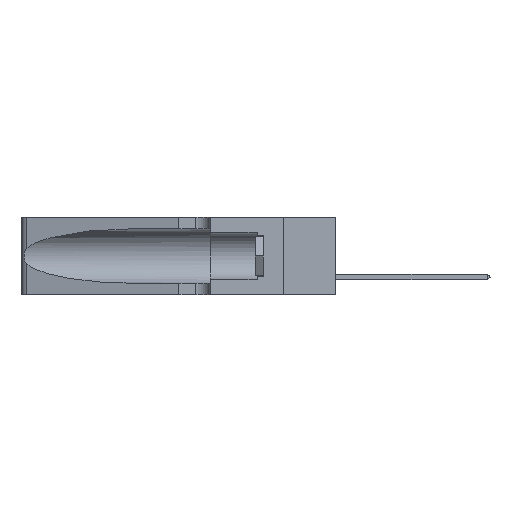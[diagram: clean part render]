
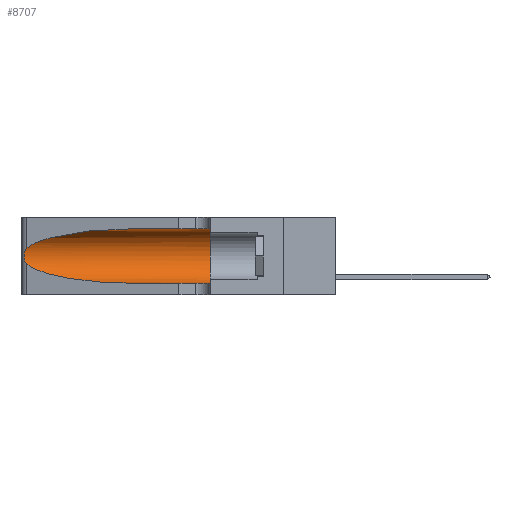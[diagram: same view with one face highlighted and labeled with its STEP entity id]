
A CAD part, left-side view. The second image highlights one B-rep face of the part: STEP entity #8707.
In plain terms, the highlighted cylindrical face has radius 3.308 mm (diameter 6.617 mm), a partial arc.
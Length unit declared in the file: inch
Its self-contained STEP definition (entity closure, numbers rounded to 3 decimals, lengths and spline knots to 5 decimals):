
#660 = EDGE_CURVE ( 'NONE', #13352, #8975, #31442, .T. ) ;
#993 = CARTESIAN_POINT ( 'NONE',  ( 0.25789, 1.23486, 0.15765 ) ) ;
#1196 = EDGE_CURVE ( 'NONE', #33338, #35989, #2201, .T. ) ;
#2098 = CARTESIAN_POINT ( 'NONE',  ( 0.25487, 1.22718, 0.22369 ) ) ;
#2140 = DIRECTION ( 'NONE',  ( 0., 0., -1. ) ) ;
#2201 =( BOUNDED_CURVE ( )  B_SPLINE_CURVE ( 3, ( #18790, #30585, #4797, #10540 ),
 .UNSPECIFIED., .F., .F. ) 
 B_SPLINE_CURVE_WITH_KNOTS ( ( 4, 4 ),
 ( 1.5708, 2.84003 ),
 .UNSPECIFIED. ) 
 CURVE ( )  GEOMETRIC_REPRESENTATION_ITEM ( )  RATIONAL_B_SPLINE_CURVE ( ( 1., 0.87, 0.87, 1. ) ) 
 REPRESENTATION_ITEM ( '' )  );
#2909 = CARTESIAN_POINT ( 'NONE',  ( 0.25487, 1.22718, 0.14631 ) ) ;
#3874 = DIRECTION ( 'NONE',  ( 0., -1., 0. ) ) ;
#4797 = CARTESIAN_POINT ( 'NONE',  ( 0.2373, 1.15595, 0.28018 ) ) ;
#5353 = CARTESIAN_POINT ( 'NONE',  ( 0.1305, 0.35, 0.185 ) ) ;
#6869 = CARTESIAN_POINT ( 'NONE',  ( 0.25639, 1.23186, 0.15144 ) ) ;
#6908 = VECTOR ( 'NONE', #3874, 39.37008 ) ;
#7624 = CARTESIAN_POINT ( 'NONE',  ( 0.1305, 1.61858, 0.185 ) ) ;
#8354 = CARTESIAN_POINT ( 'NONE',  ( 0.1305, 0.35, 0.31525 ) ) ;
#8707 = ADVANCED_FACE ( 'NONE', ( #20931 ), #25402, .F. ) ;
#8975 = VERTEX_POINT ( 'NONE', #16014 ) ;
#10086 = CARTESIAN_POINT ( 'NONE',  ( 0.26075, 1.23896, 0.19203 ) ) ;
#10387 = VERTEX_POINT ( 'NONE', #24492 ) ;
#10540 = CARTESIAN_POINT ( 'NONE',  ( 0.25487, 1.22718, 0.22369 ) ) ;
#12461 =( BOUNDED_CURVE ( )  B_SPLINE_CURVE ( 3, ( #2909, #19543, #14164, #17141 ),
 .UNSPECIFIED., .F., .T. ) 
 B_SPLINE_CURVE_WITH_KNOTS ( ( 4, 4 ),
 ( 3.44316, 4.71239 ),
 .UNSPECIFIED. ) 
 CURVE ( )  GEOMETRIC_REPRESENTATION_ITEM ( )  RATIONAL_B_SPLINE_CURVE ( ( 1., 0.87, 0.87, 1. ) ) 
 REPRESENTATION_ITEM ( '' )  );
#12479 = CARTESIAN_POINT ( 'NONE',  ( 0.25639, 1.23184, 0.21858 ) ) ;
#12591 = LINE ( 'NONE', #23389, #27291 ) ;
#12749 = CARTESIAN_POINT ( 'NONE',  ( 0.1305, 1.61858, 0.31525 ) ) ;
#12853 = CARTESIAN_POINT ( 'NONE',  ( 0.25487, 1.22718, 0.22369 ) ) ;
#12978 = CARTESIAN_POINT ( 'NONE',  ( 0.26017, 1.23833, 0.17102 ) ) ;
#13092 = ORIENTED_EDGE ( 'NONE', *, *, #27038, .T. ) ;
#13352 = VERTEX_POINT ( 'NONE', #8354 ) ;
#13659 = EDGE_CURVE ( 'NONE', #33338, #13352, #21161, .T. ) ;
#14137 = ORIENTED_EDGE ( 'NONE', *, *, #13659, .F. ) ;
#14164 = CARTESIAN_POINT ( 'NONE',  ( 0.18966, 0.96281, 0.05475 ) ) ;
#14201 = EDGE_LOOP ( 'NONE', ( #35877, #17277, #14448, #13092, #15100, #14137 ) ) ;
#14448 = ORIENTED_EDGE ( 'NONE', *, *, #26340, .T. ) ;
#15100 = ORIENTED_EDGE ( 'NONE', *, *, #660, .F. ) ;
#15360 = CARTESIAN_POINT ( 'NONE',  ( 0.25555, 1.22993, 0.14849 ) ) ;
#15850 = CARTESIAN_POINT ( 'NONE',  ( 0.25856, 1.23593, 0.16098 ) ) ;
#16014 = CARTESIAN_POINT ( 'NONE',  ( 0.1305, 0.35, 0.05475 ) ) ;
#16930 = VERTEX_POINT ( 'NONE', #29397 ) ;
#17141 = CARTESIAN_POINT ( 'NONE',  ( 0.1305, 0.72297, 0.05475 ) ) ;
#17277 = ORIENTED_EDGE ( 'NONE', *, *, #31993, .T. ) ;
#18606 = CARTESIAN_POINT ( 'NONE',  ( 0.25555, 1.22994, 0.2215 ) ) ;
#18790 = CARTESIAN_POINT ( 'NONE',  ( 0.1305, 0.72297, 0.31525 ) ) ;
#19246 = DIRECTION ( 'NONE',  ( 0., -1., 0. ) ) ;
#19543 = CARTESIAN_POINT ( 'NONE',  ( 0.2373, 1.15595, 0.08982 ) ) ;
#20931 = FACE_OUTER_BOUND ( 'NONE', #14201, .T. ) ;
#21161 = LINE ( 'NONE', #12749, #6908 ) ;
#23389 = CARTESIAN_POINT ( 'NONE',  ( 0.1305, 1.61858, 0.05475 ) ) ;
#23821 = CARTESIAN_POINT ( 'NONE',  ( 0.25854, 1.2359, 0.20912 ) ) ;
#23948 = CARTESIAN_POINT ( 'NONE',  ( 0.26018, 1.23835, 0.19895 ) ) ;
#24320 = CARTESIAN_POINT ( 'NONE',  ( 0.25787, 1.23484, 0.2124 ) ) ;
#24492 = CARTESIAN_POINT ( 'NONE',  ( 0.1305, 0.72297, 0.05475 ) ) ;
#25402 = CYLINDRICAL_SURFACE ( 'NONE', #29969, 0.13025 ) ;
#26145 = DIRECTION ( 'NONE',  ( 0., -1., 0. ) ) ;
#26340 = EDGE_CURVE ( 'NONE', #16930, #10387, #12461, .T. ) ;
#26827 = CARTESIAN_POINT ( 'NONE',  ( 0.25487, 1.22718, 0.14631 ) ) ;
#27038 = EDGE_CURVE ( 'NONE', #10387, #8975, #12591, .T. ) ;
#27291 = VECTOR ( 'NONE', #26145, 39.37008 ) ;
#28171 = DIRECTION ( 'NONE',  ( 0., 1., 0. ) ) ;
#29114 = CARTESIAN_POINT ( 'NONE',  ( 0.1305, 0.72297, 0.31525 ) ) ;
#29397 = CARTESIAN_POINT ( 'NONE',  ( 0.25487, 1.22718, 0.14631 ) ) ;
#29969 = AXIS2_PLACEMENT_3D ( 'NONE', #7624, #19246, #2140 ) ;
#30029 = CARTESIAN_POINT ( 'NONE',  ( 0.26075, 1.23896, 0.178 ) ) ;
#30585 = CARTESIAN_POINT ( 'NONE',  ( 0.18966, 0.96281, 0.31525 ) ) ;
#30755 = DIRECTION ( 'NONE',  ( 0., 0., 1. ) ) ;
#31442 = CIRCLE ( 'NONE', #31684, 0.13025 ) ;
#31684 = AXIS2_PLACEMENT_3D ( 'NONE', #5353, #28171, #30755 ) ;
#31993 = EDGE_CURVE ( 'NONE', #35989, #16930, #32749, .T. ) ;
#32749 = B_SPLINE_CURVE_WITH_KNOTS ( 'NONE', 3,
 ( #12853, #18606, #12479, #24320, #23821, #23948, #10086, #30029, #12978, #15850, #993, #6869, #15360, #26827 ),
 .UNSPECIFIED., .F., .F.,
 ( 4, 2, 2, 2, 2, 2, 4 ),
 ( 0., 0.00027, 0.00053, 0.00107, 0.0016, 0.00187, 0.00214 ),
 .UNSPECIFIED. ) ;
#33338 = VERTEX_POINT ( 'NONE', #29114 ) ;
#35877 = ORIENTED_EDGE ( 'NONE', *, *, #1196, .T. ) ;
#35989 = VERTEX_POINT ( 'NONE', #2098 ) ;
